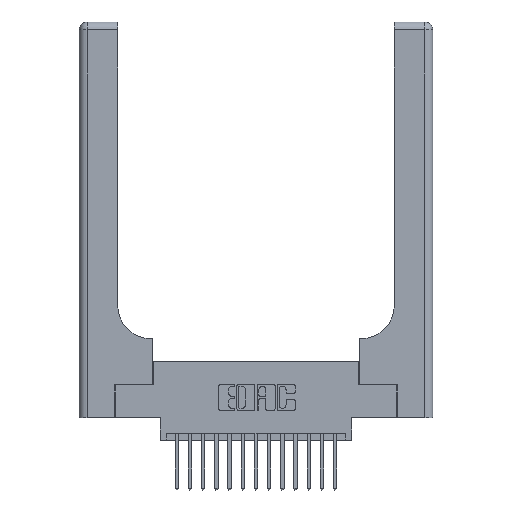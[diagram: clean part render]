
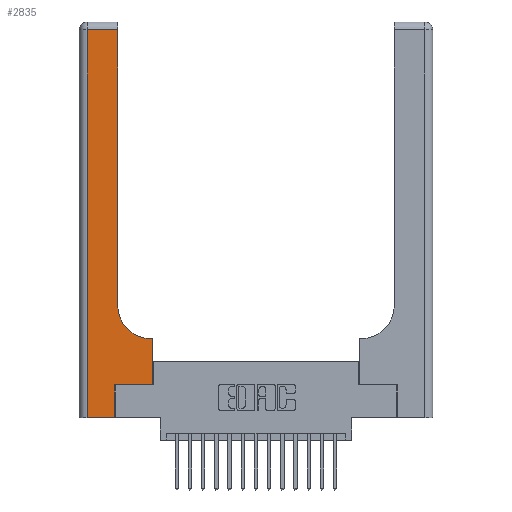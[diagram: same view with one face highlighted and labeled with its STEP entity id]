
A CAD part, top view. The second image highlights one B-rep face of the part: STEP entity #2835.
In plain terms, the highlighted planar face has unit normal (0, 0, 1).
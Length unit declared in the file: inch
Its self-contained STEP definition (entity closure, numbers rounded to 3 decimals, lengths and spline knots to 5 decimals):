
#450 = LINE ( 'NONE', #11718, #11599 ) ;
#728 = DIRECTION ( 'NONE',  ( 1., 0., 0. ) ) ;
#835 = EDGE_CURVE ( 'NONE', #4732, #11921, #14803, .T. ) ;
#1314 = DIRECTION ( 'NONE',  ( 0., -1., 0. ) ) ;
#1391 = VERTEX_POINT ( 'NONE', #2924 ) ;
#1989 = DIRECTION ( 'NONE',  ( -1., 0., 0. ) ) ;
#1992 = CARTESIAN_POINT ( 'NONE',  ( 0.5585, 0.25, 0.37 ) ) ;
#2326 = ORIENTED_EDGE ( 'NONE', *, *, #5887, .T. ) ;
#2367 = LINE ( 'NONE', #6843, #5895 ) ;
#2835 = ADVANCED_FACE ( 'NONE', ( #8262 ), #12328, .F. ) ;
#2924 = CARTESIAN_POINT ( 'NONE',  ( 0.06, 0., 0.37 ) ) ;
#3049 = ORIENTED_EDGE ( 'NONE', *, *, #14805, .T. ) ;
#3591 = CARTESIAN_POINT ( 'NONE',  ( 0., 0., 0.37 ) ) ;
#4046 = AXIS2_PLACEMENT_3D ( 'NONE', #5649, #16007, #7156 ) ;
#4732 = VERTEX_POINT ( 'NONE', #1992 ) ;
#4996 = VECTOR ( 'NONE', #1314, 39.37008 ) ;
#5134 = VECTOR ( 'NONE', #17768, 39.37008 ) ;
#5382 = CARTESIAN_POINT ( 'NONE',  ( 0.269, 0., 0.37 ) ) ;
#5649 = CARTESIAN_POINT ( 'NONE',  ( 0.5415, 0.85, 0.37 ) ) ;
#5742 = EDGE_CURVE ( 'NONE', #1391, #18634, #15786, .T. ) ;
#5887 = EDGE_CURVE ( 'NONE', #18317, #11159, #9056, .T. ) ;
#5895 = VECTOR ( 'NONE', #728, 39.37008 ) ;
#6171 = CARTESIAN_POINT ( 'NONE',  ( 0.5585, 0.6, 0.37 ) ) ;
#6344 = ORIENTED_EDGE ( 'NONE', *, *, #10664, .T. ) ;
#6744 = CARTESIAN_POINT ( 'NONE',  ( 0.2915, 3., 0.37 ) ) ;
#6843 = CARTESIAN_POINT ( 'NONE',  ( 0.269, 0.25, 0.37 ) ) ;
#7156 = DIRECTION ( 'NONE',  ( 1., 0., 0. ) ) ;
#7399 = CARTESIAN_POINT ( 'NONE',  ( 0., 2.94, 0.37 ) ) ;
#7625 = CARTESIAN_POINT ( 'NONE',  ( 0.5585, 0.25, 0.37 ) ) ;
#7680 = DIRECTION ( 'NONE',  ( 0., 1., 0. ) ) ;
#7934 = VECTOR ( 'NONE', #12487, 39.37008 ) ;
#8188 = ORIENTED_EDGE ( 'NONE', *, *, #10202, .T. ) ;
#8262 = FACE_OUTER_BOUND ( 'NONE', #18730, .T. ) ;
#8412 = ORIENTED_EDGE ( 'NONE', *, *, #16671, .T. ) ;
#8489 = CARTESIAN_POINT ( 'NONE',  ( 0.269, 0.25, 0.37 ) ) ;
#8697 = VECTOR ( 'NONE', #12666, 39.37008 ) ;
#9056 = LINE ( 'NONE', #7399, #5134 ) ;
#9810 = CARTESIAN_POINT ( 'NONE',  ( 0.06, 2.94, 0.37 ) ) ;
#9957 = EDGE_CURVE ( 'NONE', #12815, #18317, #12629, .T. ) ;
#10033 = VERTEX_POINT ( 'NONE', #17346 ) ;
#10202 = EDGE_CURVE ( 'NONE', #11159, #1391, #17279, .T. ) ;
#10664 = EDGE_CURVE ( 'NONE', #17048, #4732, #2367, .T. ) ;
#10918 = DIRECTION ( 'NONE',  ( 0., 0., -1. ) ) ;
#10944 = CARTESIAN_POINT ( 'NONE',  ( 0.2915, 0.6, 0.37 ) ) ;
#11159 = VERTEX_POINT ( 'NONE', #9810 ) ;
#11599 = VECTOR ( 'NONE', #19123, 39.37008 ) ;
#11718 = CARTESIAN_POINT ( 'NONE',  ( 0.269, 0., 0.37 ) ) ;
#11743 = CARTESIAN_POINT ( 'NONE',  ( 0.06, 3., 0.37 ) ) ;
#11921 = VERTEX_POINT ( 'NONE', #6171 ) ;
#12328 = PLANE ( 'NONE',  #13748 ) ;
#12487 = DIRECTION ( 'NONE',  ( 1., 0., 0. ) ) ;
#12629 = LINE ( 'NONE', #6744, #8697 ) ;
#12666 = DIRECTION ( 'NONE',  ( 0., 1., 0. ) ) ;
#12815 = VERTEX_POINT ( 'NONE', #15715 ) ;
#13243 = ORIENTED_EDGE ( 'NONE', *, *, #9957, .T. ) ;
#13748 = AXIS2_PLACEMENT_3D ( 'NONE', #18345, #10918, #1989 ) ;
#13946 = ORIENTED_EDGE ( 'NONE', *, *, #5742, .T. ) ;
#14803 = LINE ( 'NONE', #7625, #18332 ) ;
#14805 = EDGE_CURVE ( 'NONE', #10033, #12815, #18664, .T. ) ;
#15139 = LINE ( 'NONE', #10944, #18646 ) ;
#15268 = EDGE_CURVE ( 'NONE', #11921, #10033, #15139, .T. ) ;
#15418 = DIRECTION ( 'NONE',  ( -1., 0., 0. ) ) ;
#15715 = CARTESIAN_POINT ( 'NONE',  ( 0.2915, 0.85, 0.37 ) ) ;
#15786 = LINE ( 'NONE', #3591, #7934 ) ;
#16007 = DIRECTION ( 'NONE',  ( 0., 0., -1. ) ) ;
#16133 = CARTESIAN_POINT ( 'NONE',  ( 0.2915, 2.94, 0.37 ) ) ;
#16529 = ORIENTED_EDGE ( 'NONE', *, *, #15268, .T. ) ;
#16671 = EDGE_CURVE ( 'NONE', #18634, #17048, #450, .T. ) ;
#17016 = ORIENTED_EDGE ( 'NONE', *, *, #835, .T. ) ;
#17048 = VERTEX_POINT ( 'NONE', #8489 ) ;
#17279 = LINE ( 'NONE', #11743, #4996 ) ;
#17346 = CARTESIAN_POINT ( 'NONE',  ( 0.5415, 0.6, 0.37 ) ) ;
#17768 = DIRECTION ( 'NONE',  ( -1., 0., 0. ) ) ;
#18317 = VERTEX_POINT ( 'NONE', #16133 ) ;
#18332 = VECTOR ( 'NONE', #7680, 39.37008 ) ;
#18345 = CARTESIAN_POINT ( 'NONE',  ( 0., 3., 0.37 ) ) ;
#18634 = VERTEX_POINT ( 'NONE', #5382 ) ;
#18646 = VECTOR ( 'NONE', #15418, 39.37008 ) ;
#18664 = CIRCLE ( 'NONE', #4046, 0.25 ) ;
#18730 = EDGE_LOOP ( 'NONE', ( #13243, #2326, #8188, #13946, #8412, #6344, #17016, #16529, #3049 ) ) ;
#19123 = DIRECTION ( 'NONE',  ( 0., 1., 0. ) ) ;
